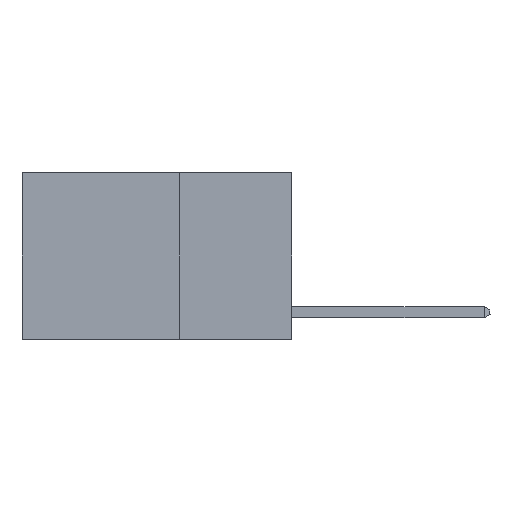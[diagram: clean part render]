
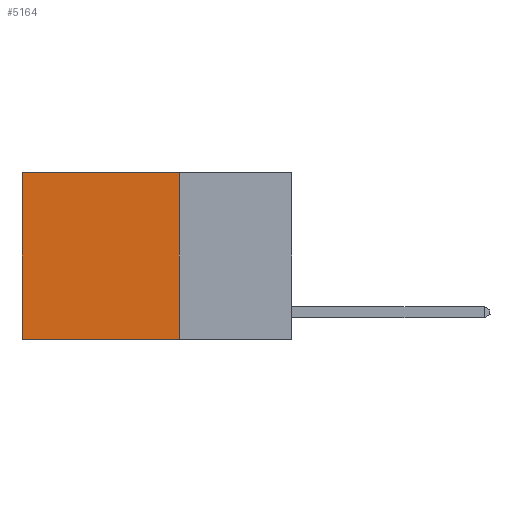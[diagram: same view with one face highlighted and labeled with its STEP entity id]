
A CAD part, left-side view. The second image highlights one B-rep face of the part: STEP entity #5164.
In plain terms, the highlighted planar face has unit normal (-1, 0, 0).
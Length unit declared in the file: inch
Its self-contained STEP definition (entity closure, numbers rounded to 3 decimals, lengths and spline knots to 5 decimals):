
#134 = DIRECTION ( 'NONE',  ( 0., 1., 0. ) ) ;
#475 = CARTESIAN_POINT ( 'NONE',  ( 0.2625, 0.6, 0. ) ) ;
#581 = VECTOR ( 'NONE', #8133, 39.37008 ) ;
#807 = CARTESIAN_POINT ( 'NONE',  ( 0.2625, 0.25, 0. ) ) ;
#968 = CARTESIAN_POINT ( 'NONE',  ( 0.2625, 0.6, 0. ) ) ;
#1102 = EDGE_CURVE ( 'NONE', #5034, #8617, #6487, .T. ) ;
#1733 = LINE ( 'NONE', #968, #2368 ) ;
#2368 = VECTOR ( 'NONE', #5509, 39.37008 ) ;
#2687 = ORIENTED_EDGE ( 'NONE', *, *, #6058, .T. ) ;
#2738 = CARTESIAN_POINT ( 'NONE',  ( 0.2625, 0.25, -0.37 ) ) ;
#2740 = CARTESIAN_POINT ( 'NONE',  ( 0.2625, 0.25, 0. ) ) ;
#2842 = CARTESIAN_POINT ( 'NONE',  ( 0.2625, 0.25, 0. ) ) ;
#2887 = FACE_OUTER_BOUND ( 'NONE', #3033, .T. ) ;
#3033 = EDGE_LOOP ( 'NONE', ( #9781, #8494, #8076, #2687 ) ) ;
#3243 = VERTEX_POINT ( 'NONE', #475 ) ;
#3331 = VECTOR ( 'NONE', #134, 39.37008 ) ;
#3642 = DIRECTION ( 'NONE',  ( 0., 1., 0. ) ) ;
#4912 = CARTESIAN_POINT ( 'NONE',  ( 0.2625, 0.6, -0.37 ) ) ;
#5034 = VERTEX_POINT ( 'NONE', #2738 ) ;
#5164 = ADVANCED_FACE ( 'NONE', ( #2887 ), #6117, .F. ) ;
#5509 = DIRECTION ( 'NONE',  ( 0., 0., -1. ) ) ;
#5573 = VECTOR ( 'NONE', #3642, 39.37008 ) ;
#6058 = EDGE_CURVE ( 'NONE', #9636, #3243, #7356, .T. ) ;
#6117 = PLANE ( 'NONE',  #6404 ) ;
#6404 = AXIS2_PLACEMENT_3D ( 'NONE', #2842, #8680, #7898 ) ;
#6487 = LINE ( 'NONE', #6788, #5573 ) ;
#6788 = CARTESIAN_POINT ( 'NONE',  ( 0.2625, 0.25, -0.37 ) ) ;
#7356 = LINE ( 'NONE', #807, #3331 ) ;
#7898 = DIRECTION ( 'NONE',  ( 0., 0., -1. ) ) ;
#8076 = ORIENTED_EDGE ( 'NONE', *, *, #9657, .F. ) ;
#8133 = DIRECTION ( 'NONE',  ( 0., 0., -1. ) ) ;
#8494 = ORIENTED_EDGE ( 'NONE', *, *, #1102, .F. ) ;
#8617 = VERTEX_POINT ( 'NONE', #4912 ) ;
#8680 = DIRECTION ( 'NONE',  ( 1., 0., 0. ) ) ;
#9307 = EDGE_CURVE ( 'NONE', #3243, #8617, #1733, .T. ) ;
#9582 = LINE ( 'NONE', #2740, #581 ) ;
#9636 = VERTEX_POINT ( 'NONE', #9692 ) ;
#9657 = EDGE_CURVE ( 'NONE', #9636, #5034, #9582, .T. ) ;
#9692 = CARTESIAN_POINT ( 'NONE',  ( 0.2625, 0.25, 0. ) ) ;
#9781 = ORIENTED_EDGE ( 'NONE', *, *, #9307, .T. ) ;
